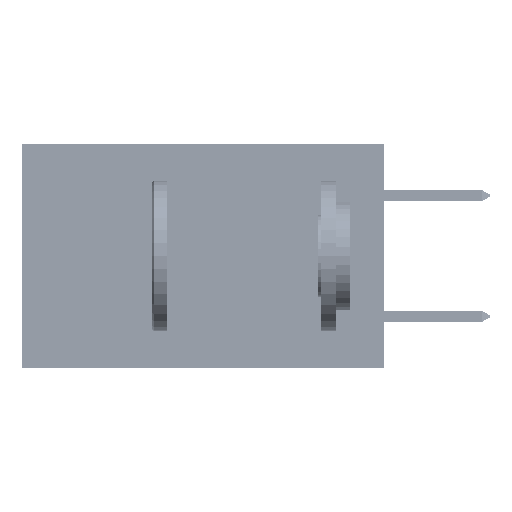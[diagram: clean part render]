
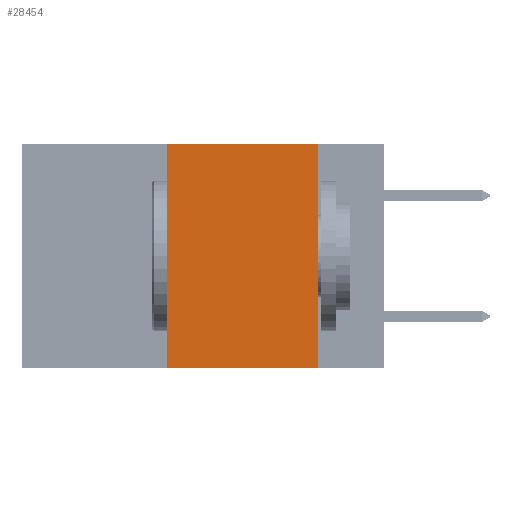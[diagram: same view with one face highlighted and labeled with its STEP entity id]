
A CAD part, left-side view. The second image highlights one B-rep face of the part: STEP entity #28454.
In plain terms, the highlighted planar face has unit normal (-1, 0, 0).
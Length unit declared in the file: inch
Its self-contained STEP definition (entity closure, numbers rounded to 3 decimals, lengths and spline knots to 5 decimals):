
#945 = CARTESIAN_POINT ( 'NONE',  ( 0., 0.11, 0. ) ) ;
#1542 = PLANE ( 'NONE',  #25565 ) ;
#1655 = VECTOR ( 'NONE', #10260, 39.37008 ) ;
#1667 = VERTEX_POINT ( 'NONE', #38368 ) ;
#3430 = LINE ( 'NONE', #945, #16447 ) ;
#4449 = ORIENTED_EDGE ( 'NONE', *, *, #14946, .T. ) ;
#5844 = ORIENTED_EDGE ( 'NONE', *, *, #13783, .F. ) ;
#8769 = CARTESIAN_POINT ( 'NONE',  ( 0., 0.11, -0.37 ) ) ;
#9506 = DIRECTION ( 'NONE',  ( 0., 0., -1. ) ) ;
#10260 = DIRECTION ( 'NONE',  ( 0., -1., 0. ) ) ;
#10314 = ORIENTED_EDGE ( 'NONE', *, *, #19867, .F. ) ;
#12026 = EDGE_LOOP ( 'NONE', ( #10314, #41028, #5844, #4449 ) ) ;
#13713 = CARTESIAN_POINT ( 'NONE',  ( 0., 0.6, 0. ) ) ;
#13783 = EDGE_CURVE ( 'NONE', #41364, #19702, #34215, .T. ) ;
#14267 = VECTOR ( 'NONE', #23524, 39.37008 ) ;
#14946 = EDGE_CURVE ( 'NONE', #41364, #29570, #42879, .T. ) ;
#16035 = CARTESIAN_POINT ( 'NONE',  ( 0., 0.6, -0.37 ) ) ;
#16447 = VECTOR ( 'NONE', #48686, 39.37008 ) ;
#17498 = CARTESIAN_POINT ( 'NONE',  ( 0., 0.36, 0. ) ) ;
#19702 = VERTEX_POINT ( 'NONE', #24578 ) ;
#19867 = EDGE_CURVE ( 'NONE', #1667, #29570, #3430, .T. ) ;
#23524 = DIRECTION ( 'NONE',  ( 0., -1., 0. ) ) ;
#24578 = CARTESIAN_POINT ( 'NONE',  ( 0., 0.36, 0. ) ) ;
#25565 = AXIS2_PLACEMENT_3D ( 'NONE', #29301, #33275, #9506 ) ;
#28454 = ADVANCED_FACE ( 'NONE', ( #35370 ), #1542, .F. ) ;
#28994 = LINE ( 'NONE', #13713, #1655 ) ;
#29301 = CARTESIAN_POINT ( 'NONE',  ( 0., 0.6, 0. ) ) ;
#29505 = DIRECTION ( 'NONE',  ( 0., 0., 1. ) ) ;
#29570 = VERTEX_POINT ( 'NONE', #8769 ) ;
#32982 = VECTOR ( 'NONE', #29505, 39.37008 ) ;
#33275 = DIRECTION ( 'NONE',  ( 1., 0., 0. ) ) ;
#34215 = LINE ( 'NONE', #17498, #32982 ) ;
#35370 = FACE_OUTER_BOUND ( 'NONE', #12026, .T. ) ;
#38368 = CARTESIAN_POINT ( 'NONE',  ( 0., 0.11, 0. ) ) ;
#41028 = ORIENTED_EDGE ( 'NONE', *, *, #50597, .F. ) ;
#41364 = VERTEX_POINT ( 'NONE', #44393 ) ;
#42879 = LINE ( 'NONE', #16035, #14267 ) ;
#44393 = CARTESIAN_POINT ( 'NONE',  ( 0., 0.36, -0.37 ) ) ;
#48686 = DIRECTION ( 'NONE',  ( 0., 0., -1. ) ) ;
#50597 = EDGE_CURVE ( 'NONE', #19702, #1667, #28994, .T. ) ;
